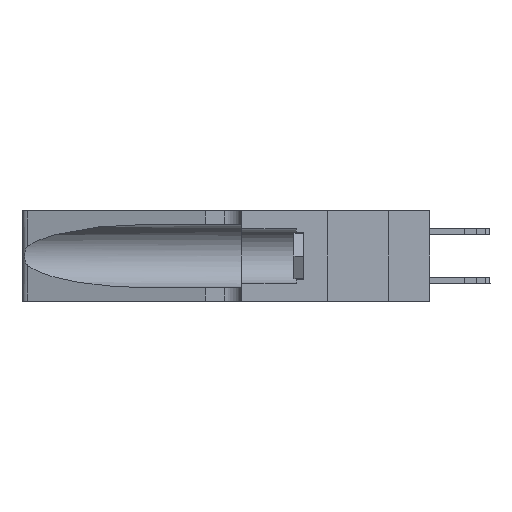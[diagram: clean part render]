
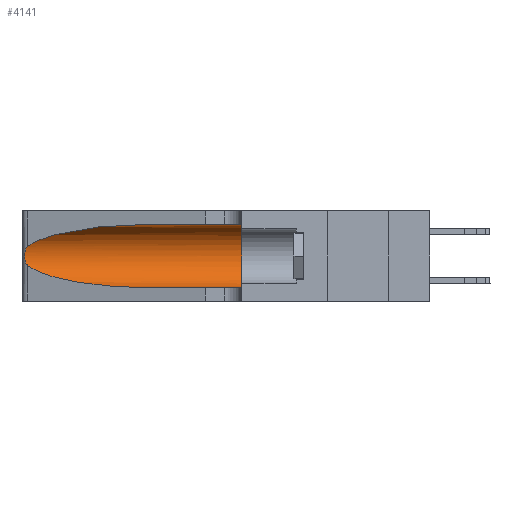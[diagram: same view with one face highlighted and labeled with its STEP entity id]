
A CAD part, left-side view. The second image highlights one B-rep face of the part: STEP entity #4141.
In plain terms, the highlighted cylindrical face has radius 3.308 mm (diameter 6.617 mm), a partial arc.
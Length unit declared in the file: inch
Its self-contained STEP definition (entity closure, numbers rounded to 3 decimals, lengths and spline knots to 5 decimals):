
#49 = ORIENTED_EDGE ( 'NONE', *, *, #18977, .T. ) ;
#310 = CARTESIAN_POINT ( 'NONE',  ( 0.26075, 1.23896, 0.19203 ) ) ;
#496 = CARTESIAN_POINT ( 'NONE',  ( 0.25639, 1.23184, 0.21858 ) ) ;
#588 = CARTESIAN_POINT ( 'NONE',  ( 0.26017, 1.23833, 0.17102 ) ) ;
#919 = CARTESIAN_POINT ( 'NONE',  ( 0.2373, 1.15595, 0.08982 ) ) ;
#1177 = LINE ( 'NONE', #26392, #15712 ) ;
#1790 = CIRCLE ( 'NONE', #20555, 0.13025 ) ;
#2608 = DIRECTION ( 'NONE',  ( 0., -1., 0. ) ) ;
#2981 = CARTESIAN_POINT ( 'NONE',  ( 0.25487, 1.22718, 0.14631 ) ) ;
#3046 = B_SPLINE_CURVE_WITH_KNOTS ( 'NONE', 3,
 ( #4479, #6716, #496, #4771, #18191, #22857, #310, #26920, #588, #9568, #25096, #11423, #4860, #22760 ),
 .UNSPECIFIED., .F., .F.,
 ( 4, 2, 2, 2, 2, 2, 4 ),
 ( 0., 0.00027, 0.00053, 0.00107, 0.0016, 0.00187, 0.00214 ),
 .UNSPECIFIED. ) ;
#4141 = ADVANCED_FACE ( 'NONE', ( #15363 ), #9477, .F. ) ;
#4205 = CARTESIAN_POINT ( 'NONE',  ( 0.1305, 0.72297, 0.31525 ) ) ;
#4309 = CARTESIAN_POINT ( 'NONE',  ( 0.25487, 1.22718, 0.22369 ) ) ;
#4479 = CARTESIAN_POINT ( 'NONE',  ( 0.25487, 1.22718, 0.22369 ) ) ;
#4771 = CARTESIAN_POINT ( 'NONE',  ( 0.25787, 1.23484, 0.2124 ) ) ;
#4860 = CARTESIAN_POINT ( 'NONE',  ( 0.25555, 1.22993, 0.14849 ) ) ;
#5479 = CARTESIAN_POINT ( 'NONE',  ( 0.1305, 0.72297, 0.31525 ) ) ;
#5532 = DIRECTION ( 'NONE',  ( 0., 1., 0. ) ) ;
#5554 = EDGE_CURVE ( 'NONE', #26229, #24165, #1790, .T. ) ;
#6716 = CARTESIAN_POINT ( 'NONE',  ( 0.25555, 1.22994, 0.2215 ) ) ;
#8089 = ORIENTED_EDGE ( 'NONE', *, *, #12320, .T. ) ;
#8873 = ORIENTED_EDGE ( 'NONE', *, *, #26462, .F. ) ;
#9234 = VERTEX_POINT ( 'NONE', #2981 ) ;
#9477 = CYLINDRICAL_SURFACE ( 'NONE', #21097, 0.13025 ) ;
#9511 = CARTESIAN_POINT ( 'NONE',  ( 0.1305, 0.72297, 0.05475 ) ) ;
#9568 = CARTESIAN_POINT ( 'NONE',  ( 0.25856, 1.23593, 0.16098 ) ) ;
#9857 = CARTESIAN_POINT ( 'NONE',  ( 0.1305, 1.61858, 0.185 ) ) ;
#11198 =( BOUNDED_CURVE ( )  B_SPLINE_CURVE ( 3, ( #4205, #26766, #17558, #4309 ),
 .UNSPECIFIED., .F., .T. ) 
 B_SPLINE_CURVE_WITH_KNOTS ( ( 4, 4 ),
 ( 1.5708, 2.84003 ),
 .UNSPECIFIED. ) 
 CURVE ( )  GEOMETRIC_REPRESENTATION_ITEM ( )  RATIONAL_B_SPLINE_CURVE ( ( 1., 0.87, 0.87, 1. ) ) 
 REPRESENTATION_ITEM ( '' )  );
#11423 = CARTESIAN_POINT ( 'NONE',  ( 0.25639, 1.23186, 0.15144 ) ) ;
#11715 = ORIENTED_EDGE ( 'NONE', *, *, #23990, .T. ) ;
#12051 = ORIENTED_EDGE ( 'NONE', *, *, #16984, .T. ) ;
#12320 = EDGE_CURVE ( 'NONE', #27853, #9234, #3046, .T. ) ;
#13749 = VECTOR ( 'NONE', #2608, 39.37008 ) ;
#13811 = CARTESIAN_POINT ( 'NONE',  ( 0.1305, 0.35, 0.185 ) ) ;
#13857 = CARTESIAN_POINT ( 'NONE',  ( 0.18966, 0.96281, 0.05475 ) ) ;
#14075 = CARTESIAN_POINT ( 'NONE',  ( 0.1305, 1.61858, 0.05475 ) ) ;
#14434 = LINE ( 'NONE', #14075, #13749 ) ;
#14474 = DIRECTION ( 'NONE',  ( 0., 0., -1. ) ) ;
#15363 = FACE_OUTER_BOUND ( 'NONE', #21640, .T. ) ;
#15712 = VECTOR ( 'NONE', #20647, 39.37008 ) ;
#16625 = DIRECTION ( 'NONE',  ( 0., 0., 1. ) ) ;
#16800 = CARTESIAN_POINT ( 'NONE',  ( 0.1305, 0.35, 0.31525 ) ) ;
#16984 = EDGE_CURVE ( 'NONE', #24825, #27853, #11198, .T. ) ;
#17558 = CARTESIAN_POINT ( 'NONE',  ( 0.2373, 1.15595, 0.28018 ) ) ;
#18191 = CARTESIAN_POINT ( 'NONE',  ( 0.25854, 1.2359, 0.20912 ) ) ;
#18588 = CARTESIAN_POINT ( 'NONE',  ( 0.25487, 1.22718, 0.22369 ) ) ;
#18977 = EDGE_CURVE ( 'NONE', #9234, #25948, #19355, .T. ) ;
#19355 =( BOUNDED_CURVE ( )  B_SPLINE_CURVE ( 3, ( #27140, #919, #13857, #9511 ),
 .UNSPECIFIED., .F., .F. ) 
 B_SPLINE_CURVE_WITH_KNOTS ( ( 4, 4 ),
 ( 3.44316, 4.71239 ),
 .UNSPECIFIED. ) 
 CURVE ( )  GEOMETRIC_REPRESENTATION_ITEM ( )  RATIONAL_B_SPLINE_CURVE ( ( 1., 0.87, 0.87, 1. ) ) 
 REPRESENTATION_ITEM ( '' )  );
#20555 = AXIS2_PLACEMENT_3D ( 'NONE', #13811, #5532, #16625 ) ;
#20647 = DIRECTION ( 'NONE',  ( 0., -1., 0. ) ) ;
#21097 = AXIS2_PLACEMENT_3D ( 'NONE', #9857, #23445, #14474 ) ;
#21465 = ORIENTED_EDGE ( 'NONE', *, *, #5554, .F. ) ;
#21640 = EDGE_LOOP ( 'NONE', ( #12051, #8089, #49, #11715, #21465, #8873 ) ) ;
#22760 = CARTESIAN_POINT ( 'NONE',  ( 0.25487, 1.22718, 0.14631 ) ) ;
#22857 = CARTESIAN_POINT ( 'NONE',  ( 0.26018, 1.23835, 0.19895 ) ) ;
#23130 = CARTESIAN_POINT ( 'NONE',  ( 0.1305, 0.35, 0.05475 ) ) ;
#23445 = DIRECTION ( 'NONE',  ( 0., -1., 0. ) ) ;
#23990 = EDGE_CURVE ( 'NONE', #25948, #24165, #14434, .T. ) ;
#24165 = VERTEX_POINT ( 'NONE', #23130 ) ;
#24825 = VERTEX_POINT ( 'NONE', #5479 ) ;
#25066 = CARTESIAN_POINT ( 'NONE',  ( 0.1305, 0.72297, 0.05475 ) ) ;
#25096 = CARTESIAN_POINT ( 'NONE',  ( 0.25789, 1.23486, 0.15765 ) ) ;
#25948 = VERTEX_POINT ( 'NONE', #25066 ) ;
#26229 = VERTEX_POINT ( 'NONE', #16800 ) ;
#26392 = CARTESIAN_POINT ( 'NONE',  ( 0.1305, 1.61858, 0.31525 ) ) ;
#26462 = EDGE_CURVE ( 'NONE', #24825, #26229, #1177, .T. ) ;
#26766 = CARTESIAN_POINT ( 'NONE',  ( 0.18966, 0.96281, 0.31525 ) ) ;
#26920 = CARTESIAN_POINT ( 'NONE',  ( 0.26075, 1.23896, 0.178 ) ) ;
#27140 = CARTESIAN_POINT ( 'NONE',  ( 0.25487, 1.22718, 0.14631 ) ) ;
#27853 = VERTEX_POINT ( 'NONE', #18588 ) ;
